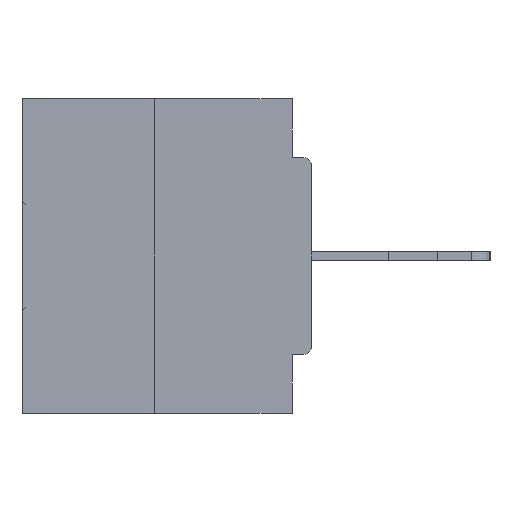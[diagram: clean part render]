
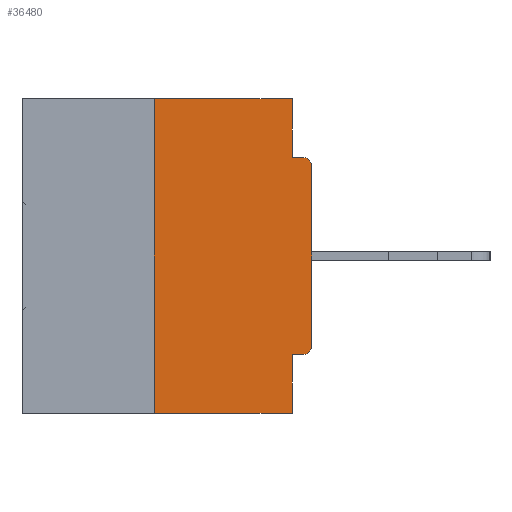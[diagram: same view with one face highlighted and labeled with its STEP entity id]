
A CAD part, left-side view. The second image highlights one B-rep face of the part: STEP entity #36480.
In plain terms, the highlighted planar face has unit normal (-1, 0, 0).
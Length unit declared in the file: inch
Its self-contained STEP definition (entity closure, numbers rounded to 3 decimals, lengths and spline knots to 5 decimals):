
#982 = AXIS2_PLACEMENT_3D ( 'NONE', #14696, #2445, #23159 ) ;
#1253 = PLANE ( 'NONE',  #982 ) ;
#2120 = CARTESIAN_POINT ( 'NONE',  ( 0., 0.015, -0.1085 ) ) ;
#2445 = DIRECTION ( 'NONE',  ( 1., 0., 0. ) ) ;
#2968 = CARTESIAN_POINT ( 'NONE',  ( 0., 0., -0.1085 ) ) ;
#3184 = ORIENTED_EDGE ( 'NONE', *, *, #37106, .T. ) ;
#3912 = AXIS2_PLACEMENT_3D ( 'NONE', #2120, #35074, #35851 ) ;
#3995 = EDGE_CURVE ( 'NONE', #39345, #37613, #27491, .T. ) ;
#4358 = CARTESIAN_POINT ( 'NONE',  ( 0., 0.015, -0.3915 ) ) ;
#4550 = DIRECTION ( 'NONE',  ( -1., 0., 0. ) ) ;
#6958 = EDGE_CURVE ( 'NONE', #14088, #15948, #20593, .T. ) ;
#8059 = CARTESIAN_POINT ( 'NONE',  ( 0., 0.031, -0.4065 ) ) ;
#8375 = VECTOR ( 'NONE', #36092, 39.37008 ) ;
#8662 = DIRECTION ( 'NONE',  ( 0., -1., 0. ) ) ;
#8987 = CARTESIAN_POINT ( 'NONE',  ( 0., 0., 0. ) ) ;
#10196 = AXIS2_PLACEMENT_3D ( 'NONE', #4358, #4550, #28824 ) ;
#10824 = ORIENTED_EDGE ( 'NONE', *, *, #39530, .F. ) ;
#10947 = CARTESIAN_POINT ( 'NONE',  ( 0., 0.25, -0.5 ) ) ;
#11877 = ORIENTED_EDGE ( 'NONE', *, *, #38239, .F. ) ;
#11909 = VECTOR ( 'NONE', #16084, 39.37008 ) ;
#11985 = VECTOR ( 'NONE', #31806, 39.37008 ) ;
#12413 = CARTESIAN_POINT ( 'NONE',  ( 0., 0., -0.3915 ) ) ;
#13403 = ORIENTED_EDGE ( 'NONE', *, *, #25032, .T. ) ;
#14088 = VERTEX_POINT ( 'NONE', #2968 ) ;
#14141 = EDGE_CURVE ( 'NONE', #35097, #15948, #33279, .T. ) ;
#14498 = CARTESIAN_POINT ( 'NONE',  ( 0., 0.031, 0. ) ) ;
#14693 = EDGE_CURVE ( 'NONE', #25350, #30440, #16504, .T. ) ;
#14696 = CARTESIAN_POINT ( 'NONE',  ( 0., 0.46, 0. ) ) ;
#15948 = VERTEX_POINT ( 'NONE', #37254 ) ;
#16084 = DIRECTION ( 'NONE',  ( 0., 0., -1. ) ) ;
#16504 = LINE ( 'NONE', #34770, #36090 ) ;
#16672 = LINE ( 'NONE', #28530, #30123 ) ;
#16905 = EDGE_LOOP ( 'NONE', ( #22203, #21529, #3184, #10824, #19167, #17029, #13403, #30944, #31480, #11877 ) ) ;
#17029 = ORIENTED_EDGE ( 'NONE', *, *, #3995, .T. ) ;
#17313 = CARTESIAN_POINT ( 'NONE',  ( 0., 0.25, 0. ) ) ;
#17756 = CARTESIAN_POINT ( 'NONE',  ( 0., 0., -0.4065 ) ) ;
#19167 = ORIENTED_EDGE ( 'NONE', *, *, #28218, .F. ) ;
#20593 = CIRCLE ( 'NONE', #3912, 0.015 ) ;
#21088 = LINE ( 'NONE', #33740, #22740 ) ;
#21529 = ORIENTED_EDGE ( 'NONE', *, *, #24447, .F. ) ;
#21555 = VERTEX_POINT ( 'NONE', #10947 ) ;
#22203 = ORIENTED_EDGE ( 'NONE', *, *, #14693, .F. ) ;
#22732 = LINE ( 'NONE', #25525, #11909 ) ;
#22740 = VECTOR ( 'NONE', #8662, 39.37008 ) ;
#23159 = DIRECTION ( 'NONE',  ( 0., 0., -1. ) ) ;
#23874 = VECTOR ( 'NONE', #36105, 39.37008 ) ;
#24447 = EDGE_CURVE ( 'NONE', #21555, #25350, #16672, .T. ) ;
#25032 = EDGE_CURVE ( 'NONE', #37613, #14088, #39317, .T. ) ;
#25350 = VERTEX_POINT ( 'NONE', #17313 ) ;
#25525 = CARTESIAN_POINT ( 'NONE',  ( 0., 0.031, 0. ) ) ;
#27445 = CARTESIAN_POINT ( 'NONE',  ( 0., 0., -0.0935 ) ) ;
#27491 = CIRCLE ( 'NONE', #10196, 0.015 ) ;
#27994 = CARTESIAN_POINT ( 'NONE',  ( 0., 0.031, -0.5 ) ) ;
#28218 = EDGE_CURVE ( 'NONE', #39345, #37001, #33021, .T. ) ;
#28530 = CARTESIAN_POINT ( 'NONE',  ( 0., 0.25, 0. ) ) ;
#28625 = VERTEX_POINT ( 'NONE', #38947 ) ;
#28768 = FACE_OUTER_BOUND ( 'NONE', #16905, .T. ) ;
#28824 = DIRECTION ( 'NONE',  ( 0., 0., -1. ) ) ;
#28910 = DIRECTION ( 'NONE',  ( 0., 0., 1. ) ) ;
#30123 = VECTOR ( 'NONE', #28910, 39.37008 ) ;
#30440 = VERTEX_POINT ( 'NONE', #14498 ) ;
#30803 = CARTESIAN_POINT ( 'NONE',  ( 0., 0.015, -0.4065 ) ) ;
#30944 = ORIENTED_EDGE ( 'NONE', *, *, #6958, .T. ) ;
#31004 = CARTESIAN_POINT ( 'NONE',  ( 0., 0.031, -0.0935 ) ) ;
#31480 = ORIENTED_EDGE ( 'NONE', *, *, #14141, .F. ) ;
#31806 = DIRECTION ( 'NONE',  ( 0., 0., -1. ) ) ;
#32599 = DIRECTION ( 'NONE',  ( 0., 1., 0. ) ) ;
#33021 = LINE ( 'NONE', #17756, #37452 ) ;
#33279 = LINE ( 'NONE', #27445, #23874 ) ;
#33740 = CARTESIAN_POINT ( 'NONE',  ( 0., 0.46, -0.5 ) ) ;
#34567 = DIRECTION ( 'NONE',  ( 0., -1., 0. ) ) ;
#34770 = CARTESIAN_POINT ( 'NONE',  ( 0., 0.46, 0. ) ) ;
#35074 = DIRECTION ( 'NONE',  ( -1., 0., 0. ) ) ;
#35097 = VERTEX_POINT ( 'NONE', #31004 ) ;
#35851 = DIRECTION ( 'NONE',  ( 0., 0., -1. ) ) ;
#36090 = VECTOR ( 'NONE', #34567, 39.37008 ) ;
#36092 = DIRECTION ( 'NONE',  ( 0., 0., 1. ) ) ;
#36105 = DIRECTION ( 'NONE',  ( 0., -1., 0. ) ) ;
#36480 = ADVANCED_FACE ( 'NONE', ( #28768 ), #1253, .F. ) ;
#37001 = VERTEX_POINT ( 'NONE', #8059 ) ;
#37106 = EDGE_CURVE ( 'NONE', #21555, #28625, #21088, .T. ) ;
#37254 = CARTESIAN_POINT ( 'NONE',  ( 0., 0.015, -0.0935 ) ) ;
#37452 = VECTOR ( 'NONE', #32599, 39.37008 ) ;
#37613 = VERTEX_POINT ( 'NONE', #12413 ) ;
#37637 = LINE ( 'NONE', #27994, #11985 ) ;
#38239 = EDGE_CURVE ( 'NONE', #30440, #35097, #22732, .T. ) ;
#38947 = CARTESIAN_POINT ( 'NONE',  ( 0., 0.031, -0.5 ) ) ;
#39317 = LINE ( 'NONE', #8987, #8375 ) ;
#39345 = VERTEX_POINT ( 'NONE', #30803 ) ;
#39530 = EDGE_CURVE ( 'NONE', #37001, #28625, #37637, .T. ) ;
